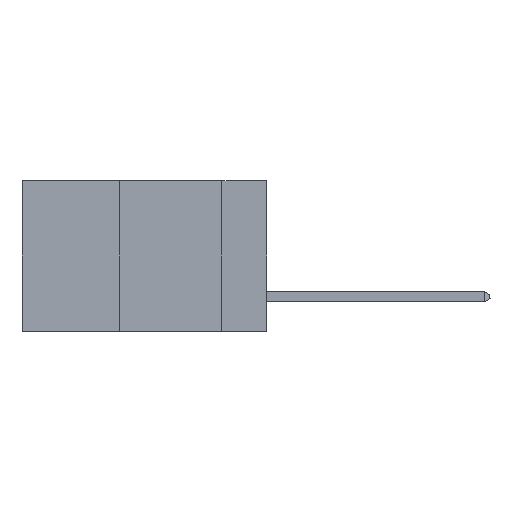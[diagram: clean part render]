
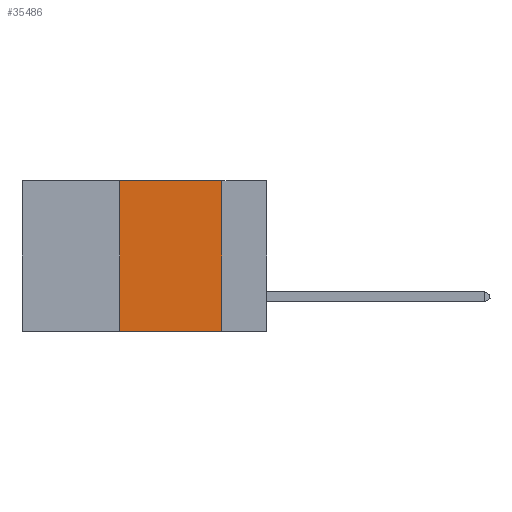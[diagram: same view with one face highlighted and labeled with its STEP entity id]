
A CAD part, left-side view. The second image highlights one B-rep face of the part: STEP entity #35486.
In plain terms, the highlighted planar face has unit normal (-1, 0, 0).
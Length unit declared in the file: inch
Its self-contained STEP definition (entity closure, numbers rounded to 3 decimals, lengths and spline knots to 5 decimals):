
#386 = CARTESIAN_POINT ( 'NONE',  ( 0., 0.36, -0.37 ) ) ;
#2642 = VECTOR ( 'NONE', #32213, 39.37008 ) ;
#3387 = CARTESIAN_POINT ( 'NONE',  ( 0., 0.36, 0. ) ) ;
#4124 = VERTEX_POINT ( 'NONE', #29904 ) ;
#4981 = DIRECTION ( 'NONE',  ( 0., 0., 1. ) ) ;
#5110 = CARTESIAN_POINT ( 'NONE',  ( 0., 0.6, 0. ) ) ;
#5271 = DIRECTION ( 'NONE',  ( 1., 0., 0. ) ) ;
#5716 = LINE ( 'NONE', #21871, #15074 ) ;
#6494 = EDGE_CURVE ( 'NONE', #4124, #8389, #16662, .T. ) ;
#8389 = VERTEX_POINT ( 'NONE', #45982 ) ;
#8838 = DIRECTION ( 'NONE',  ( 0., 0., -1. ) ) ;
#9215 = ORIENTED_EDGE ( 'NONE', *, *, #6494, .F. ) ;
#10711 = DIRECTION ( 'NONE',  ( 0., -1., 0. ) ) ;
#10953 = ORIENTED_EDGE ( 'NONE', *, *, #43710, .F. ) ;
#11942 = EDGE_CURVE ( 'NONE', #25360, #8389, #15804, .T. ) ;
#15074 = VECTOR ( 'NONE', #10711, 39.37008 ) ;
#15804 = LINE ( 'NONE', #38905, #36350 ) ;
#16096 = VECTOR ( 'NONE', #4981, 39.37008 ) ;
#16662 = LINE ( 'NONE', #39725, #2642 ) ;
#19287 = ORIENTED_EDGE ( 'NONE', *, *, #47030, .F. ) ;
#20038 = CARTESIAN_POINT ( 'NONE',  ( 0., 0.36, 0. ) ) ;
#21871 = CARTESIAN_POINT ( 'NONE',  ( 0., 0.6, 0. ) ) ;
#25225 = VERTEX_POINT ( 'NONE', #3387 ) ;
#25360 = VERTEX_POINT ( 'NONE', #386 ) ;
#25476 = FACE_OUTER_BOUND ( 'NONE', #37856, .T. ) ;
#25603 = ORIENTED_EDGE ( 'NONE', *, *, #11942, .T. ) ;
#29904 = CARTESIAN_POINT ( 'NONE',  ( 0., 0.11, 0. ) ) ;
#32213 = DIRECTION ( 'NONE',  ( 0., 0., -1. ) ) ;
#35317 = DIRECTION ( 'NONE',  ( 0., -1., 0. ) ) ;
#35486 = ADVANCED_FACE ( 'NONE', ( #25476 ), #46184, .F. ) ;
#36350 = VECTOR ( 'NONE', #35317, 39.37008 ) ;
#37856 = EDGE_LOOP ( 'NONE', ( #9215, #19287, #10953, #25603 ) ) ;
#38905 = CARTESIAN_POINT ( 'NONE',  ( 0., 0.6, -0.37 ) ) ;
#39725 = CARTESIAN_POINT ( 'NONE',  ( 0., 0.11, 0. ) ) ;
#42264 = AXIS2_PLACEMENT_3D ( 'NONE', #5110, #5271, #8838 ) ;
#43710 = EDGE_CURVE ( 'NONE', #25360, #25225, #47150, .T. ) ;
#45982 = CARTESIAN_POINT ( 'NONE',  ( 0., 0.11, -0.37 ) ) ;
#46184 = PLANE ( 'NONE',  #42264 ) ;
#47030 = EDGE_CURVE ( 'NONE', #25225, #4124, #5716, .T. ) ;
#47150 = LINE ( 'NONE', #20038, #16096 ) ;
